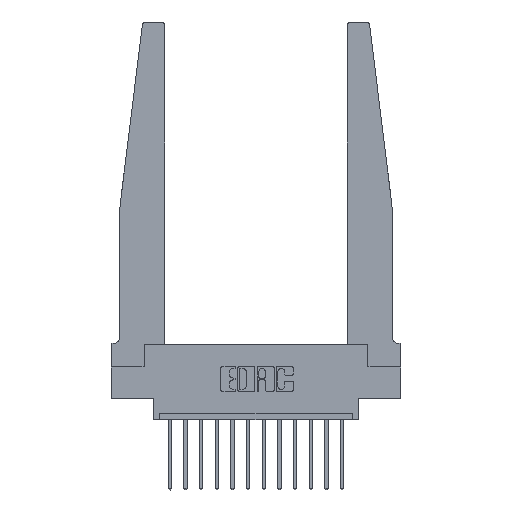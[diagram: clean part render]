
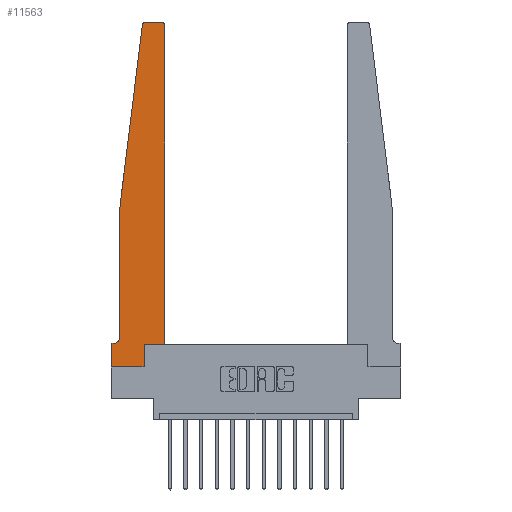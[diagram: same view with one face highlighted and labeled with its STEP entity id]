
A CAD part, top view. The second image highlights one B-rep face of the part: STEP entity #11563.
In plain terms, the highlighted planar face has unit normal (0, 0, 1).
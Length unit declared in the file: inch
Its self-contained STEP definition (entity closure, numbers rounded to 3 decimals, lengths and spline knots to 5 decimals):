
#101 = CIRCLE ( 'NONE', #12793, 0.03 ) ;
#399 = DIRECTION ( 'NONE',  ( -0.122, -0.992, 0. ) ) ;
#548 = ORIENTED_EDGE ( 'NONE', *, *, #6662, .T. ) ;
#742 = LINE ( 'NONE', #5179, #13333 ) ;
#1070 = CARTESIAN_POINT ( 'NONE',  ( 0.065, 0.2375, 0.37 ) ) ;
#1133 = LINE ( 'NONE', #5489, #9426 ) ;
#1257 = ORIENTED_EDGE ( 'NONE', *, *, #2206, .T. ) ;
#1467 = VERTEX_POINT ( 'NONE', #1724 ) ;
#1667 = VECTOR ( 'NONE', #399, 39.37008 ) ;
#1724 = CARTESIAN_POINT ( 'NONE',  ( 0., 0.1875, 0.37 ) ) ;
#1801 = AXIS2_PLACEMENT_3D ( 'NONE', #3348, #14745, #5861 ) ;
#2035 = CARTESIAN_POINT ( 'NONE',  ( 0.395, 2.75, 0.37 ) ) ;
#2088 = PLANE ( 'NONE',  #13710 ) ;
#2206 = EDGE_CURVE ( 'NONE', #12129, #6280, #1133, .T. ) ;
#2261 = CARTESIAN_POINT ( 'NONE',  ( 0., 0.1875, 0.37 ) ) ;
#2637 = EDGE_CURVE ( 'NONE', #13563, #12073, #742, .T. ) ;
#2807 = VERTEX_POINT ( 'NONE', #2035 ) ;
#2818 = CARTESIAN_POINT ( 'NONE',  ( 0.065, 0.1875, 0.37 ) ) ;
#2863 = CARTESIAN_POINT ( 'NONE',  ( 0.065, 1.25, 0.37 ) ) ;
#2914 = LINE ( 'NONE', #13072, #9603 ) ;
#2920 = CARTESIAN_POINT ( 'NONE',  ( 0.27653, 2.72, 0.37 ) ) ;
#2931 = EDGE_LOOP ( 'NONE', ( #5485, #10455, #548, #3134, #5571, #15589, #8834, #1257, #4519, #8341, #4313, #10840 ) ) ;
#3134 = ORIENTED_EDGE ( 'NONE', *, *, #2637, .T. ) ;
#3348 = CARTESIAN_POINT ( 'NONE',  ( 0.015, 0.2375, 0.37 ) ) ;
#3568 = VERTEX_POINT ( 'NONE', #14144 ) ;
#3774 = VERTEX_POINT ( 'NONE', #10798 ) ;
#3926 = LINE ( 'NONE', #15209, #12590 ) ;
#4169 = EDGE_CURVE ( 'NONE', #1467, #12129, #12116, .T. ) ;
#4279 = AXIS2_PLACEMENT_3D ( 'NONE', #7720, #9034, #7666 ) ;
#4313 = ORIENTED_EDGE ( 'NONE', *, *, #16275, .T. ) ;
#4314 = CARTESIAN_POINT ( 'NONE',  ( 0.425, 0.18, 0.37 ) ) ;
#4519 = ORIENTED_EDGE ( 'NONE', *, *, #14980, .T. ) ;
#4799 = DIRECTION ( 'NONE',  ( 1., 0., 0. ) ) ;
#5143 = CARTESIAN_POINT ( 'NONE',  ( 0.25, 2.75, 0.37 ) ) ;
#5179 = CARTESIAN_POINT ( 'NONE',  ( 0.065, 1.25, 0.37 ) ) ;
#5485 = ORIENTED_EDGE ( 'NONE', *, *, #10867, .T. ) ;
#5489 = CARTESIAN_POINT ( 'NONE',  ( 0., 0., 0.37 ) ) ;
#5571 = ORIENTED_EDGE ( 'NONE', *, *, #7478, .T. ) ;
#5861 = DIRECTION ( 'NONE',  ( -1., 0., 0. ) ) ;
#5878 = FACE_OUTER_BOUND ( 'NONE', #2931, .T. ) ;
#5892 = VERTEX_POINT ( 'NONE', #10596 ) ;
#6225 = CARTESIAN_POINT ( 'NONE',  ( 0., 0., 0.37 ) ) ;
#6280 = VERTEX_POINT ( 'NONE', #8905 ) ;
#6662 = EDGE_CURVE ( 'NONE', #5892, #13563, #8747, .T. ) ;
#6753 = CARTESIAN_POINT ( 'NONE',  ( 0., 0., 0.37 ) ) ;
#7408 = DIRECTION ( 'NONE',  ( 0., 0., 1. ) ) ;
#7478 = EDGE_CURVE ( 'NONE', #12073, #13903, #10137, .T. ) ;
#7563 = DIRECTION ( 'NONE',  ( 1., 0., 0. ) ) ;
#7666 = DIRECTION ( 'NONE',  ( 1., 0., 0. ) ) ;
#7720 = CARTESIAN_POINT ( 'NONE',  ( 0.395, 2.72, 0.37 ) ) ;
#7905 = EDGE_CURVE ( 'NONE', #13903, #1467, #10948, .T. ) ;
#7923 = VERTEX_POINT ( 'NONE', #11659 ) ;
#8015 = DIRECTION ( 'NONE',  ( 0., 1., 0. ) ) ;
#8341 = ORIENTED_EDGE ( 'NONE', *, *, #10920, .T. ) ;
#8747 = LINE ( 'NONE', #2863, #1667 ) ;
#8834 = ORIENTED_EDGE ( 'NONE', *, *, #4169, .T. ) ;
#8905 = CARTESIAN_POINT ( 'NONE',  ( 0.2605, 0., 0.37 ) ) ;
#9034 = DIRECTION ( 'NONE',  ( 0., 0., 1. ) ) ;
#9058 = EDGE_CURVE ( 'NONE', #3568, #2807, #14246, .T. ) ;
#9059 = DIRECTION ( 'NONE',  ( -1., 0., 0. ) ) ;
#9306 = DIRECTION ( 'NONE',  ( 1., 0., 0. ) ) ;
#9353 = DIRECTION ( 'NONE',  ( 0., 1., 0. ) ) ;
#9426 = VECTOR ( 'NONE', #9306, 39.37008 ) ;
#9544 = CARTESIAN_POINT ( 'NONE',  ( 0.015, 0.1875, 0.37 ) ) ;
#9603 = VECTOR ( 'NONE', #9353, 39.37008 ) ;
#10137 = CIRCLE ( 'NONE', #1801, 0.05 ) ;
#10351 = VECTOR ( 'NONE', #9059, 39.37008 ) ;
#10455 = ORIENTED_EDGE ( 'NONE', *, *, #15533, .T. ) ;
#10479 = CARTESIAN_POINT ( 'NONE',  ( 0.065, 1.25, 0.37 ) ) ;
#10540 = CARTESIAN_POINT ( 'NONE',  ( 0.27653, 2.75, 0.37 ) ) ;
#10596 = CARTESIAN_POINT ( 'NONE',  ( 0.24675, 2.72367, 0.37 ) ) ;
#10798 = CARTESIAN_POINT ( 'NONE',  ( 0.2605, 0.18, 0.37 ) ) ;
#10840 = ORIENTED_EDGE ( 'NONE', *, *, #9058, .T. ) ;
#10867 = EDGE_CURVE ( 'NONE', #2807, #14555, #15401, .T. ) ;
#10920 = EDGE_CURVE ( 'NONE', #3774, #7923, #3926, .T. ) ;
#10948 = LINE ( 'NONE', #2818, #10351 ) ;
#11563 = ADVANCED_FACE ( 'NONE', ( #5878 ), #2088, .T. ) ;
#11659 = CARTESIAN_POINT ( 'NONE',  ( 0.425, 0.18, 0.37 ) ) ;
#11662 = DIRECTION ( 'NONE',  ( 0., -1., 0. ) ) ;
#11732 = VECTOR ( 'NONE', #8015, 39.37008 ) ;
#12073 = VERTEX_POINT ( 'NONE', #1070 ) ;
#12116 = LINE ( 'NONE', #6753, #15288 ) ;
#12129 = VERTEX_POINT ( 'NONE', #6225 ) ;
#12590 = VECTOR ( 'NONE', #7563, 39.37008 ) ;
#12793 = AXIS2_PLACEMENT_3D ( 'NONE', #2920, #15907, #16056 ) ;
#13072 = CARTESIAN_POINT ( 'NONE',  ( 0.2605, 0.18, 0.37 ) ) ;
#13105 = DIRECTION ( 'NONE',  ( 0., -1., 0. ) ) ;
#13333 = VECTOR ( 'NONE', #11662, 39.37008 ) ;
#13563 = VERTEX_POINT ( 'NONE', #10479 ) ;
#13710 = AXIS2_PLACEMENT_3D ( 'NONE', #2261, #7408, #4799 ) ;
#13903 = VERTEX_POINT ( 'NONE', #9544 ) ;
#13982 = VECTOR ( 'NONE', #15494, 39.37008 ) ;
#14144 = CARTESIAN_POINT ( 'NONE',  ( 0.425, 2.72, 0.37 ) ) ;
#14246 = CIRCLE ( 'NONE', #4279, 0.03 ) ;
#14555 = VERTEX_POINT ( 'NONE', #10540 ) ;
#14745 = DIRECTION ( 'NONE',  ( 0., 0., -1. ) ) ;
#14980 = EDGE_CURVE ( 'NONE', #6280, #3774, #2914, .T. ) ;
#15209 = CARTESIAN_POINT ( 'NONE',  ( 0.425, 0.18, 0.37 ) ) ;
#15288 = VECTOR ( 'NONE', #13105, 39.37008 ) ;
#15401 = LINE ( 'NONE', #5143, #13982 ) ;
#15494 = DIRECTION ( 'NONE',  ( -1., 0., 0. ) ) ;
#15533 = EDGE_CURVE ( 'NONE', #14555, #5892, #101, .T. ) ;
#15589 = ORIENTED_EDGE ( 'NONE', *, *, #7905, .T. ) ;
#15907 = DIRECTION ( 'NONE',  ( 0., 0., 1. ) ) ;
#16056 = DIRECTION ( 'NONE',  ( 1., 0., 0. ) ) ;
#16090 = LINE ( 'NONE', #4314, #11732 ) ;
#16275 = EDGE_CURVE ( 'NONE', #7923, #3568, #16090, .T. ) ;
